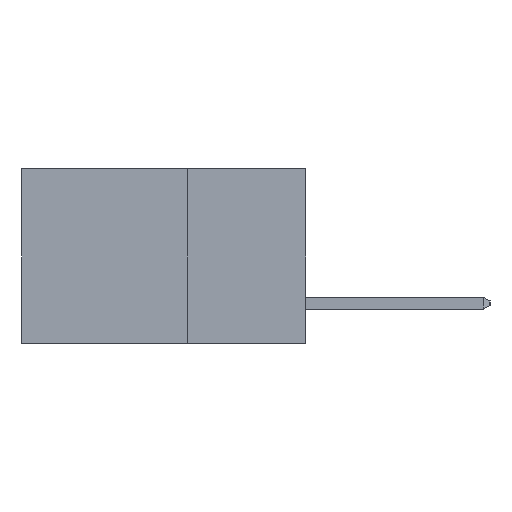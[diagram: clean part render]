
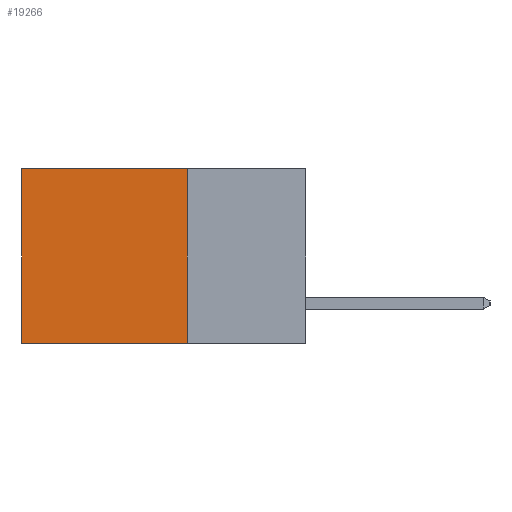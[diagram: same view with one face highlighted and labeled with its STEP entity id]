
A CAD part, left-side view. The second image highlights one B-rep face of the part: STEP entity #19266.
In plain terms, the highlighted planar face has unit normal (-1, 0, 0).
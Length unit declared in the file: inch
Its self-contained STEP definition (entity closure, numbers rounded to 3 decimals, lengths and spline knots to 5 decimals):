
#505 = EDGE_CURVE ( 'NONE', #9828, #12122, #9168, .T. ) ;
#1200 = CARTESIAN_POINT ( 'NONE',  ( 0.2615, 0.25, 0. ) ) ;
#1421 = CARTESIAN_POINT ( 'NONE',  ( 0.2615, 0.25, -0.37 ) ) ;
#1450 = VERTEX_POINT ( 'NONE', #2924 ) ;
#2150 = ORIENTED_EDGE ( 'NONE', *, *, #6935, .F. ) ;
#2763 = DIRECTION ( 'NONE',  ( 0., 0., -1. ) ) ;
#2924 = CARTESIAN_POINT ( 'NONE',  ( 0.2615, 0.6, 0. ) ) ;
#3101 = PLANE ( 'NONE',  #9020 ) ;
#3287 = ORIENTED_EDGE ( 'NONE', *, *, #6623, .T. ) ;
#4060 = VERTEX_POINT ( 'NONE', #14901 ) ;
#4645 = DIRECTION ( 'NONE',  ( 0., 0., -1. ) ) ;
#4902 = LINE ( 'NONE', #1200, #15879 ) ;
#5420 = ORIENTED_EDGE ( 'NONE', *, *, #505, .F. ) ;
#5818 = CARTESIAN_POINT ( 'NONE',  ( 0.2615, 0.25, -0.37 ) ) ;
#6020 = ORIENTED_EDGE ( 'NONE', *, *, #18854, .T. ) ;
#6570 = CARTESIAN_POINT ( 'NONE',  ( 0.2615, 0.6, -0.37 ) ) ;
#6623 = EDGE_CURVE ( 'NONE', #1450, #4060, #15690, .T. ) ;
#6935 = EDGE_CURVE ( 'NONE', #12122, #4060, #14546, .T. ) ;
#7441 = DIRECTION ( 'NONE',  ( 0., 1., 0. ) ) ;
#9020 = AXIS2_PLACEMENT_3D ( 'NONE', #12191, #13662, #4645 ) ;
#9168 = LINE ( 'NONE', #1421, #12653 ) ;
#9828 = VERTEX_POINT ( 'NONE', #18794 ) ;
#9857 = EDGE_LOOP ( 'NONE', ( #3287, #2150, #5420, #6020 ) ) ;
#10215 = FACE_OUTER_BOUND ( 'NONE', #9857, .T. ) ;
#10611 = VECTOR ( 'NONE', #18894, 39.37008 ) ;
#12122 = VERTEX_POINT ( 'NONE', #5818 ) ;
#12191 = CARTESIAN_POINT ( 'NONE',  ( 0.2615, 0.25, -0.37 ) ) ;
#12653 = VECTOR ( 'NONE', #2763, 39.37008 ) ;
#13662 = DIRECTION ( 'NONE',  ( 1., 0., 0. ) ) ;
#14546 = LINE ( 'NONE', #17537, #10611 ) ;
#14901 = CARTESIAN_POINT ( 'NONE',  ( 0.2615, 0.6, -0.37 ) ) ;
#15230 = VECTOR ( 'NONE', #15473, 39.37008 ) ;
#15473 = DIRECTION ( 'NONE',  ( 0., 0., -1. ) ) ;
#15690 = LINE ( 'NONE', #6570, #15230 ) ;
#15879 = VECTOR ( 'NONE', #7441, 39.37008 ) ;
#17537 = CARTESIAN_POINT ( 'NONE',  ( 0.2615, 0.25, -0.37 ) ) ;
#18794 = CARTESIAN_POINT ( 'NONE',  ( 0.2615, 0.25, 0. ) ) ;
#18854 = EDGE_CURVE ( 'NONE', #9828, #1450, #4902, .T. ) ;
#18894 = DIRECTION ( 'NONE',  ( 0., 1., 0. ) ) ;
#19266 = ADVANCED_FACE ( 'NONE', ( #10215 ), #3101, .F. ) ;
